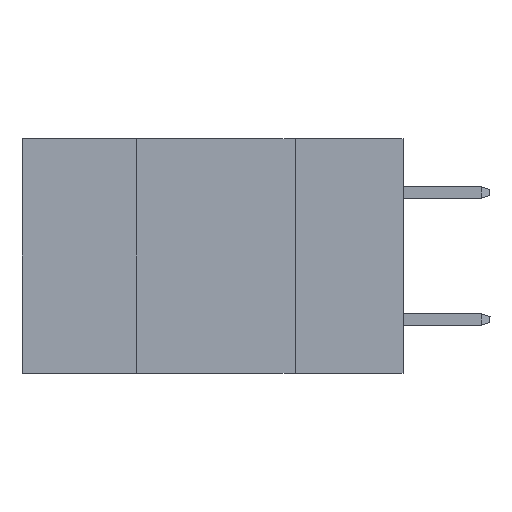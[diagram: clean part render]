
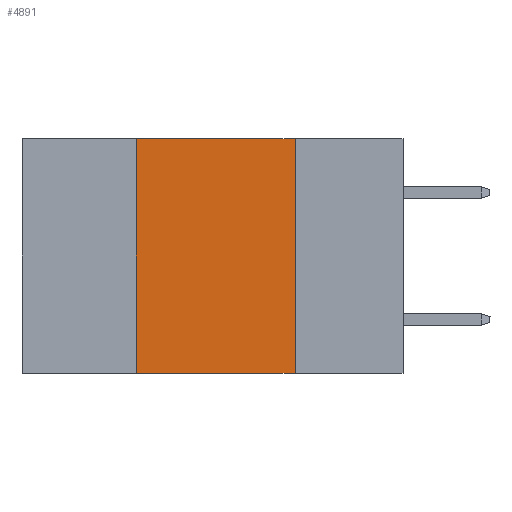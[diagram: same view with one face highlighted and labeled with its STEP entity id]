
A CAD part, left-side view. The second image highlights one B-rep face of the part: STEP entity #4891.
In plain terms, the highlighted planar face has unit normal (-1, 0, 0).
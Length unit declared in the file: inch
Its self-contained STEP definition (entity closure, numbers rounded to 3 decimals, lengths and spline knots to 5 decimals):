
#69 = VECTOR ( 'NONE', #10870, 39.37008 ) ;
#244 = VECTOR ( 'NONE', #3491, 39.37008 ) ;
#254 = CARTESIAN_POINT ( 'NONE',  ( 0., 0.6, 0. ) ) ;
#505 = LINE ( 'NONE', #8294, #6817 ) ;
#1240 = FACE_OUTER_BOUND ( 'NONE', #4222, .T. ) ;
#1336 = CARTESIAN_POINT ( 'NONE',  ( 0., 0.17, 0. ) ) ;
#1560 = DIRECTION ( 'NONE',  ( 0., 0., 1. ) ) ;
#2401 = DIRECTION ( 'NONE',  ( 1., 0., 0. ) ) ;
#2412 = LINE ( 'NONE', #3434, #13461 ) ;
#3057 = VERTEX_POINT ( 'NONE', #1336 ) ;
#3434 = CARTESIAN_POINT ( 'NONE',  ( 0., 0.42, 0. ) ) ;
#3491 = DIRECTION ( 'NONE',  ( 0., -1., 0. ) ) ;
#3637 = CARTESIAN_POINT ( 'NONE',  ( 0., 0.17, -0.37 ) ) ;
#3913 = VERTEX_POINT ( 'NONE', #7935 ) ;
#4053 = ORIENTED_EDGE ( 'NONE', *, *, #8989, .F. ) ;
#4222 = EDGE_LOOP ( 'NONE', ( #4053, #6912, #8120, #10692 ) ) ;
#4512 = VERTEX_POINT ( 'NONE', #8064 ) ;
#4891 = ADVANCED_FACE ( 'NONE', ( #1240 ), #5703, .F. ) ;
#4893 = EDGE_CURVE ( 'NONE', #3913, #3057, #9108, .T. ) ;
#5703 = PLANE ( 'NONE',  #6510 ) ;
#6439 = CARTESIAN_POINT ( 'NONE',  ( 0., 0.17, 0. ) ) ;
#6510 = AXIS2_PLACEMENT_3D ( 'NONE', #254, #2401, #10121 ) ;
#6817 = VECTOR ( 'NONE', #8561, 39.37008 ) ;
#6912 = ORIENTED_EDGE ( 'NONE', *, *, #4893, .F. ) ;
#7475 = EDGE_CURVE ( 'NONE', #4512, #3913, #2412, .T. ) ;
#7935 = CARTESIAN_POINT ( 'NONE',  ( 0., 0.42, 0. ) ) ;
#8064 = CARTESIAN_POINT ( 'NONE',  ( 0., 0.42, -0.37 ) ) ;
#8120 = ORIENTED_EDGE ( 'NONE', *, *, #7475, .F. ) ;
#8294 = CARTESIAN_POINT ( 'NONE',  ( 0., 0.6, -0.37 ) ) ;
#8561 = DIRECTION ( 'NONE',  ( 0., -1., 0. ) ) ;
#8989 = EDGE_CURVE ( 'NONE', #3057, #12930, #13030, .T. ) ;
#9108 = LINE ( 'NONE', #13448, #244 ) ;
#10121 = DIRECTION ( 'NONE',  ( 0., 0., -1. ) ) ;
#10692 = ORIENTED_EDGE ( 'NONE', *, *, #10881, .T. ) ;
#10870 = DIRECTION ( 'NONE',  ( 0., 0., -1. ) ) ;
#10881 = EDGE_CURVE ( 'NONE', #4512, #12930, #505, .T. ) ;
#12930 = VERTEX_POINT ( 'NONE', #3637 ) ;
#13030 = LINE ( 'NONE', #6439, #69 ) ;
#13448 = CARTESIAN_POINT ( 'NONE',  ( 0., 0.6, 0. ) ) ;
#13461 = VECTOR ( 'NONE', #1560, 39.37008 ) ;
